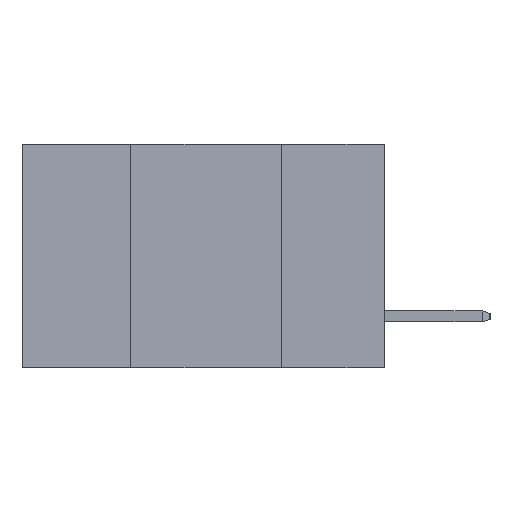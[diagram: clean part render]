
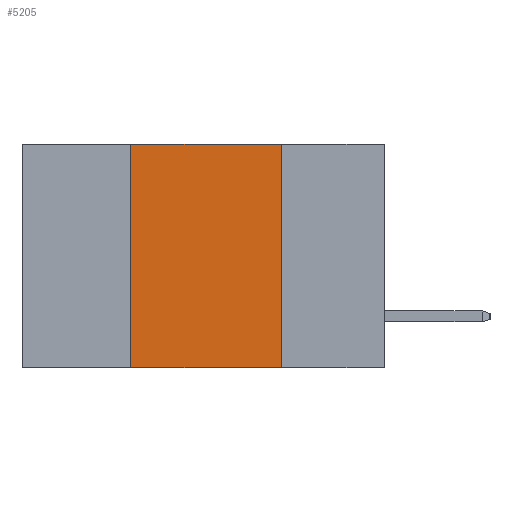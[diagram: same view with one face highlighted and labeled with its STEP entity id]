
A CAD part, left-side view. The second image highlights one B-rep face of the part: STEP entity #5205.
In plain terms, the highlighted planar face has unit normal (-1, 0, 0).
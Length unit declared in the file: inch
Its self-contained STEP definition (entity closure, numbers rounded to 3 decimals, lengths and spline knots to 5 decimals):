
#197 = CARTESIAN_POINT ( 'NONE',  ( 0., 0.42, 0. ) ) ;
#243 = VECTOR ( 'NONE', #1910, 39.37008 ) ;
#652 = EDGE_CURVE ( 'NONE', #3968, #9036, #11978, .T. ) ;
#727 = CARTESIAN_POINT ( 'NONE',  ( 0., 0.17, 0. ) ) ;
#836 = CARTESIAN_POINT ( 'NONE',  ( 0., 0.42, 0. ) ) ;
#1079 = VECTOR ( 'NONE', #10395, 39.37008 ) ;
#1117 = LINE ( 'NONE', #10575, #10207 ) ;
#1292 = ORIENTED_EDGE ( 'NONE', *, *, #652, .F. ) ;
#1315 = CARTESIAN_POINT ( 'NONE',  ( 0., 0.17, -0.37 ) ) ;
#1488 = PLANE ( 'NONE',  #4668 ) ;
#1732 = VERTEX_POINT ( 'NONE', #1315 ) ;
#1910 = DIRECTION ( 'NONE',  ( 0., 0., 1. ) ) ;
#3850 = FACE_OUTER_BOUND ( 'NONE', #4425, .T. ) ;
#3968 = VERTEX_POINT ( 'NONE', #197 ) ;
#4200 = LINE ( 'NONE', #727, #1079 ) ;
#4425 = EDGE_LOOP ( 'NONE', ( #11162, #1292, #9340, #6048 ) ) ;
#4668 = AXIS2_PLACEMENT_3D ( 'NONE', #7997, #9218, #10793 ) ;
#4842 = CARTESIAN_POINT ( 'NONE',  ( 0., 0.6, 0. ) ) ;
#5205 = ADVANCED_FACE ( 'NONE', ( #3850 ), #1488, .F. ) ;
#5775 = LINE ( 'NONE', #836, #243 ) ;
#6048 = ORIENTED_EDGE ( 'NONE', *, *, #9316, .T. ) ;
#7003 = DIRECTION ( 'NONE',  ( 0., -1., 0. ) ) ;
#7496 = CARTESIAN_POINT ( 'NONE',  ( 0., 0.17, 0. ) ) ;
#7997 = CARTESIAN_POINT ( 'NONE',  ( 0., 0.6, 0. ) ) ;
#9036 = VERTEX_POINT ( 'NONE', #7496 ) ;
#9218 = DIRECTION ( 'NONE',  ( 1., 0., 0. ) ) ;
#9316 = EDGE_CURVE ( 'NONE', #12120, #1732, #1117, .T. ) ;
#9340 = ORIENTED_EDGE ( 'NONE', *, *, #9901, .F. ) ;
#9373 = DIRECTION ( 'NONE',  ( 0., -1., 0. ) ) ;
#9694 = VECTOR ( 'NONE', #9373, 39.37008 ) ;
#9901 = EDGE_CURVE ( 'NONE', #12120, #3968, #5775, .T. ) ;
#10207 = VECTOR ( 'NONE', #7003, 39.37008 ) ;
#10395 = DIRECTION ( 'NONE',  ( 0., 0., -1. ) ) ;
#10476 = EDGE_CURVE ( 'NONE', #9036, #1732, #4200, .T. ) ;
#10575 = CARTESIAN_POINT ( 'NONE',  ( 0., 0.6, -0.37 ) ) ;
#10717 = CARTESIAN_POINT ( 'NONE',  ( 0., 0.42, -0.37 ) ) ;
#10793 = DIRECTION ( 'NONE',  ( 0., 0., -1. ) ) ;
#11162 = ORIENTED_EDGE ( 'NONE', *, *, #10476, .F. ) ;
#11978 = LINE ( 'NONE', #4842, #9694 ) ;
#12120 = VERTEX_POINT ( 'NONE', #10717 ) ;
